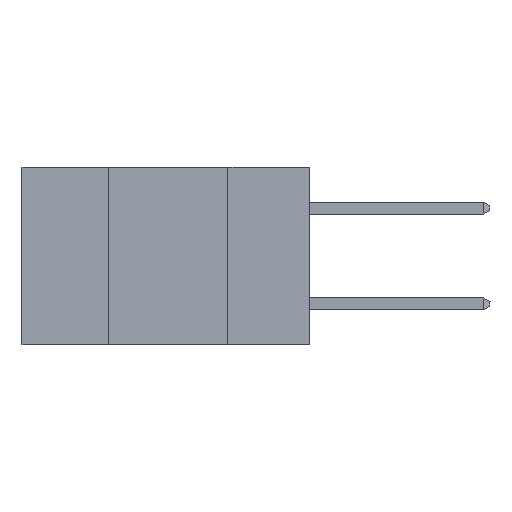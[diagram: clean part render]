
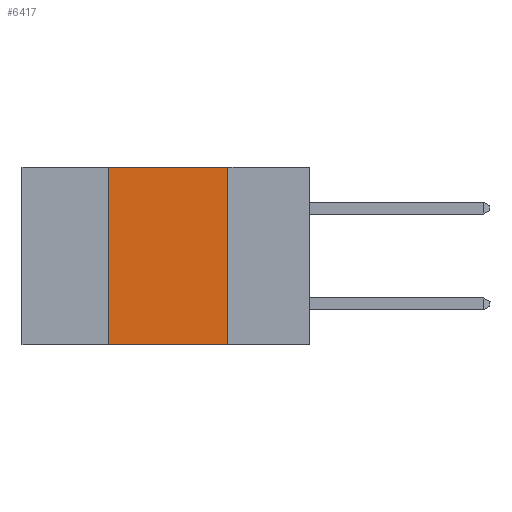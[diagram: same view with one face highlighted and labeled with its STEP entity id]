
A CAD part, left-side view. The second image highlights one B-rep face of the part: STEP entity #6417.
In plain terms, the highlighted planar face has unit normal (-1, 0, 0).
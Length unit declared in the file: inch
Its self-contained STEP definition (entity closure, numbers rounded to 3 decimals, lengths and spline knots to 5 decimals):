
#1780 = VERTEX_POINT ( 'NONE', #33163 ) ;
#1947 = CARTESIAN_POINT ( 'NONE',  ( 0., 0.17, 0. ) ) ;
#2152 = DIRECTION ( 'NONE',  ( 0., 0., -1. ) ) ;
#2253 = EDGE_CURVE ( 'NONE', #25852, #1780, #17808, .T. ) ;
#3081 = EDGE_CURVE ( 'NONE', #25852, #7909, #38514, .T. ) ;
#3423 = VECTOR ( 'NONE', #34488, 39.37008 ) ;
#5685 = FACE_OUTER_BOUND ( 'NONE', #21602, .T. ) ;
#5873 = DIRECTION ( 'NONE',  ( 1., 0., 0. ) ) ;
#6417 = ADVANCED_FACE ( 'NONE', ( #5685 ), #15609, .F. ) ;
#7779 = DIRECTION ( 'NONE',  ( 0., -1., 0. ) ) ;
#7909 = VERTEX_POINT ( 'NONE', #38298 ) ;
#7912 = CARTESIAN_POINT ( 'NONE',  ( 0., 0.6, 0. ) ) ;
#9013 = CARTESIAN_POINT ( 'NONE',  ( 0., 0.6, -0.37 ) ) ;
#9099 = CARTESIAN_POINT ( 'NONE',  ( 0., 0.42, 0. ) ) ;
#9430 = AXIS2_PLACEMENT_3D ( 'NONE', #21568, #5873, #34256 ) ;
#13168 = VERTEX_POINT ( 'NONE', #1947 ) ;
#13362 = VECTOR ( 'NONE', #15607, 39.37008 ) ;
#13926 = ORIENTED_EDGE ( 'NONE', *, *, #22473, .F. ) ;
#15607 = DIRECTION ( 'NONE',  ( 0., -1., 0. ) ) ;
#15609 = PLANE ( 'NONE',  #9430 ) ;
#17808 = LINE ( 'NONE', #9013, #13362 ) ;
#21054 = CARTESIAN_POINT ( 'NONE',  ( 0., 0.17, 0. ) ) ;
#21568 = CARTESIAN_POINT ( 'NONE',  ( 0., 0.6, 0. ) ) ;
#21602 = EDGE_LOOP ( 'NONE', ( #13926, #39336, #40600, #22211 ) ) ;
#22211 = ORIENTED_EDGE ( 'NONE', *, *, #2253, .T. ) ;
#22437 = CARTESIAN_POINT ( 'NONE',  ( 0., 0.42, -0.37 ) ) ;
#22473 = EDGE_CURVE ( 'NONE', #13168, #1780, #32532, .T. ) ;
#22963 = EDGE_CURVE ( 'NONE', #7909, #13168, #35952, .T. ) ;
#25852 = VERTEX_POINT ( 'NONE', #22437 ) ;
#29007 = VECTOR ( 'NONE', #7779, 39.37008 ) ;
#31057 = VECTOR ( 'NONE', #2152, 39.37008 ) ;
#32532 = LINE ( 'NONE', #21054, #31057 ) ;
#33163 = CARTESIAN_POINT ( 'NONE',  ( 0., 0.17, -0.37 ) ) ;
#34256 = DIRECTION ( 'NONE',  ( 0., 0., -1. ) ) ;
#34488 = DIRECTION ( 'NONE',  ( 0., 0., 1. ) ) ;
#35952 = LINE ( 'NONE', #7912, #29007 ) ;
#38298 = CARTESIAN_POINT ( 'NONE',  ( 0., 0.42, 0. ) ) ;
#38514 = LINE ( 'NONE', #9099, #3423 ) ;
#39336 = ORIENTED_EDGE ( 'NONE', *, *, #22963, .F. ) ;
#40600 = ORIENTED_EDGE ( 'NONE', *, *, #3081, .F. ) ;
